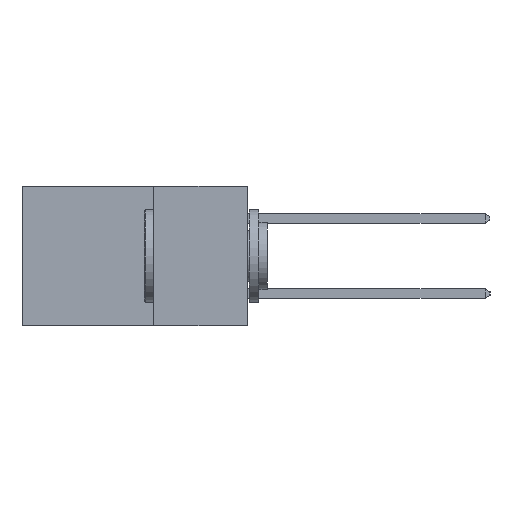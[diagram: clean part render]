
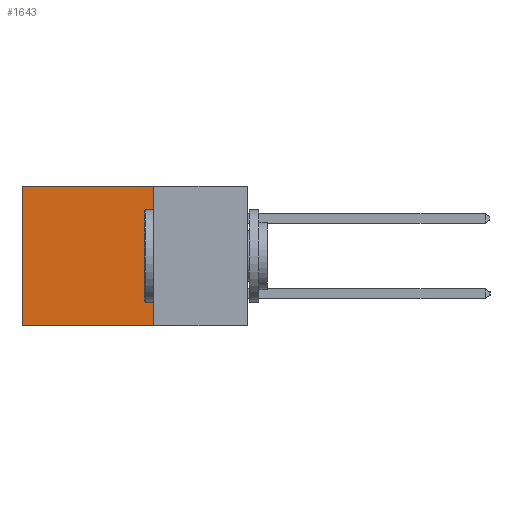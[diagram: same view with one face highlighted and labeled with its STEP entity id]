
A CAD part, left-side view. The second image highlights one B-rep face of the part: STEP entity #1643.
In plain terms, the highlighted planar face has unit normal (-1, 0, 0).
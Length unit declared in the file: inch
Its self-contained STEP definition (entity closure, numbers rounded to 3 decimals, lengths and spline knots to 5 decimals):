
#1435 = VECTOR ( 'NONE', #16632, 39.37008 ) ;
#1485 = DIRECTION ( 'NONE',  ( 0., 0., -1. ) ) ;
#1643 = ADVANCED_FACE ( 'NONE', ( #13497 ), #14980, .F. ) ;
#2328 = CARTESIAN_POINT ( 'NONE',  ( 0.2615, 0.25, -0.37 ) ) ;
#3371 = VECTOR ( 'NONE', #12171, 39.37008 ) ;
#3715 = ORIENTED_EDGE ( 'NONE', *, *, #10502, .T. ) ;
#3880 = ORIENTED_EDGE ( 'NONE', *, *, #16864, .F. ) ;
#4276 = CARTESIAN_POINT ( 'NONE',  ( 0.2615, 0.25, 0. ) ) ;
#5779 = ORIENTED_EDGE ( 'NONE', *, *, #7218, .T. ) ;
#7218 = EDGE_CURVE ( 'NONE', #16452, #19467, #7694, .T. ) ;
#7327 = DIRECTION ( 'NONE',  ( 0., 0., -1. ) ) ;
#7594 = VECTOR ( 'NONE', #1485, 39.37008 ) ;
#7694 = LINE ( 'NONE', #4276, #3371 ) ;
#8081 = CARTESIAN_POINT ( 'NONE',  ( 0.2615, 0.6, -0.37 ) ) ;
#9286 = CARTESIAN_POINT ( 'NONE',  ( 0.2615, 0.25, -0.37 ) ) ;
#9456 = EDGE_CURVE ( 'NONE', #16452, #15853, #14754, .T. ) ;
#9498 = LINE ( 'NONE', #2328, #1435 ) ;
#9631 = ORIENTED_EDGE ( 'NONE', *, *, #9456, .F. ) ;
#10224 = CARTESIAN_POINT ( 'NONE',  ( 0.2615, 0.6, 0. ) ) ;
#10502 = EDGE_CURVE ( 'NONE', #19467, #12669, #11779, .T. ) ;
#10598 = VECTOR ( 'NONE', #7327, 39.37008 ) ;
#10983 = CARTESIAN_POINT ( 'NONE',  ( 0.2615, 0.25, 0. ) ) ;
#11779 = LINE ( 'NONE', #8081, #7594 ) ;
#12171 = DIRECTION ( 'NONE',  ( 0., 1., 0. ) ) ;
#12669 = VERTEX_POINT ( 'NONE', #16243 ) ;
#13497 = FACE_OUTER_BOUND ( 'NONE', #14611, .T. ) ;
#13564 = CARTESIAN_POINT ( 'NONE',  ( 0.2615, 0.25, -0.37 ) ) ;
#14611 = EDGE_LOOP ( 'NONE', ( #3715, #3880, #9631, #5779 ) ) ;
#14754 = LINE ( 'NONE', #13564, #10598 ) ;
#14980 = PLANE ( 'NONE',  #18296 ) ;
#15853 = VERTEX_POINT ( 'NONE', #19075 ) ;
#16243 = CARTESIAN_POINT ( 'NONE',  ( 0.2615, 0.6, -0.37 ) ) ;
#16452 = VERTEX_POINT ( 'NONE', #10983 ) ;
#16632 = DIRECTION ( 'NONE',  ( 0., 1., 0. ) ) ;
#16864 = EDGE_CURVE ( 'NONE', #15853, #12669, #9498, .T. ) ;
#17113 = DIRECTION ( 'NONE',  ( 0., 0., -1. ) ) ;
#17140 = DIRECTION ( 'NONE',  ( 1., 0., 0. ) ) ;
#18296 = AXIS2_PLACEMENT_3D ( 'NONE', #9286, #17140, #17113 ) ;
#19075 = CARTESIAN_POINT ( 'NONE',  ( 0.2615, 0.25, -0.37 ) ) ;
#19467 = VERTEX_POINT ( 'NONE', #10224 ) ;
